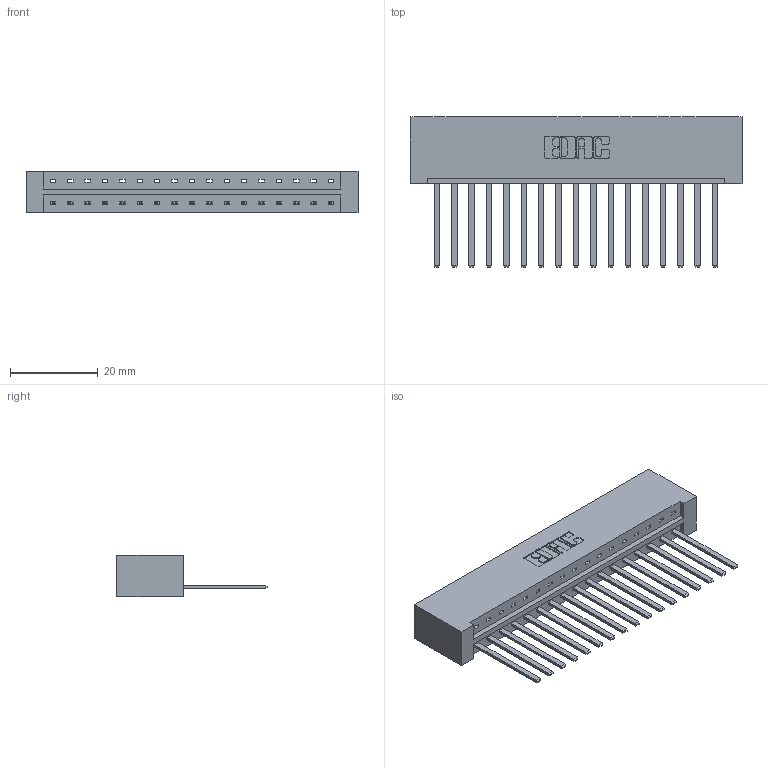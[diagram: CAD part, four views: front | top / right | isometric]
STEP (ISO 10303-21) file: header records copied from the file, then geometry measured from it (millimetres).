
FILE_DESCRIPTION (( 'STEP AP203' ), '1' );
FILE_NAME ('333-017-544-101.STEP', '2019-08-09T12:13:49', ( '' ), ( '' ), 'SwSTEP 2.0', 'SolidWorks 2016', '' );
FILE_SCHEMA (( 'CONFIG_CONTROL_DESIGN' ));
Length unit declared in the file: inch
Products named in the file (3): 345-292-001_345-293-144; 333 Part_Lugless; 333-017-544-101
Assembly tree (18 placements, depth 2):
  333-017-544-101
    333 Part_Lugless
    345-292-001_345-293-144  x17
Bounding box: 75.62 x 34.3 x 9.4 mm (x, y, z)
Volume: 8203.7 mm3; surface area: 9309.3 mm2
Topology: 18 solids, 18 shells, 990 faces, 2973 edges, 1958 vertices
Faces by surface type: plane 712, cylinder 278
Entity records: 13165 total; most frequent: CARTESIAN_POINT 2281, ORIENTED_EDGE 2234, DIRECTION 1963, EDGE_CURVE 1117, VECTOR 1001, LINE 1001, VERTEX_POINT 742, AXIS2_PLACEMENT_3D 481
